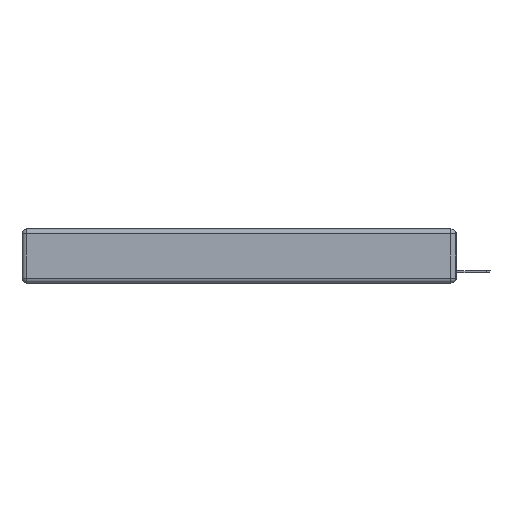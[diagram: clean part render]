
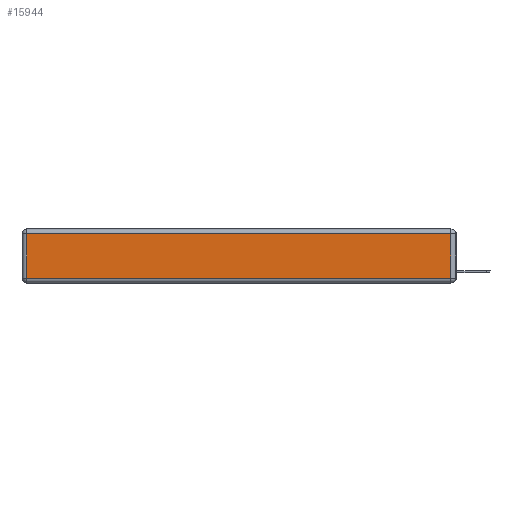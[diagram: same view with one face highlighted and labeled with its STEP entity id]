
A CAD part, left-side view. The second image highlights one B-rep face of the part: STEP entity #15944.
In plain terms, the highlighted planar face has unit normal (-1, 0, 0).
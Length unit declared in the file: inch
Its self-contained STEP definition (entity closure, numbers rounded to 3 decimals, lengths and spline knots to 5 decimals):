
#41 = CARTESIAN_POINT ( 'NONE',  ( 0., 0., -0.343 ) ) ;
#593 = LINE ( 'NONE', #10791, #13308 ) ;
#784 = VERTEX_POINT ( 'NONE', #3760 ) ;
#988 = VECTOR ( 'NONE', #2317, 39.37008 ) ;
#1004 = CARTESIAN_POINT ( 'NONE',  ( 0., 2.72, -0.343 ) ) ;
#2317 = DIRECTION ( 'NONE',  ( 0., 0., -1. ) ) ;
#2895 = EDGE_CURVE ( 'NONE', #784, #14623, #15143, .T. ) ;
#3760 = CARTESIAN_POINT ( 'NONE',  ( 0., 0.03, -0.03 ) ) ;
#4066 = CARTESIAN_POINT ( 'NONE',  ( 0., 0.03, -0.313 ) ) ;
#4266 = DIRECTION ( 'NONE',  ( 0., 0., 1. ) ) ;
#4416 = EDGE_CURVE ( 'NONE', #14623, #6491, #9836, .T. ) ;
#6491 = VERTEX_POINT ( 'NONE', #11413 ) ;
#7182 = VECTOR ( 'NONE', #13332, 39.37008 ) ;
#7221 = DIRECTION ( 'NONE',  ( 0., 0., 1. ) ) ;
#7301 = ORIENTED_EDGE ( 'NONE', *, *, #4416, .T. ) ;
#8003 = CARTESIAN_POINT ( 'NONE',  ( 0., 0.03, -0.343 ) ) ;
#8514 = PLANE ( 'NONE',  #10298 ) ;
#8618 = ORIENTED_EDGE ( 'NONE', *, *, #14991, .T. ) ;
#9686 = ORIENTED_EDGE ( 'NONE', *, *, #2895, .T. ) ;
#9836 = LINE ( 'NONE', #1004, #988 ) ;
#10298 = AXIS2_PLACEMENT_3D ( 'NONE', #41, #14648, #7221 ) ;
#10682 = DIRECTION ( 'NONE',  ( 0., -1., 0. ) ) ;
#10720 = EDGE_LOOP ( 'NONE', ( #14382, #8618, #9686, #7301 ) ) ;
#10767 = CARTESIAN_POINT ( 'NONE',  ( 0., 2.75, -0.03 ) ) ;
#10791 = CARTESIAN_POINT ( 'NONE',  ( 0., 0., -0.313 ) ) ;
#10901 = EDGE_CURVE ( 'NONE', #6491, #14197, #593, .T. ) ;
#11262 = VECTOR ( 'NONE', #4266, 39.37008 ) ;
#11413 = CARTESIAN_POINT ( 'NONE',  ( 0., 2.72, -0.313 ) ) ;
#11701 = FACE_OUTER_BOUND ( 'NONE', #10720, .T. ) ;
#13308 = VECTOR ( 'NONE', #10682, 39.37008 ) ;
#13332 = DIRECTION ( 'NONE',  ( 0., 1., 0. ) ) ;
#13600 = CARTESIAN_POINT ( 'NONE',  ( 0., 2.72, -0.03 ) ) ;
#13823 = LINE ( 'NONE', #8003, #11262 ) ;
#14197 = VERTEX_POINT ( 'NONE', #4066 ) ;
#14382 = ORIENTED_EDGE ( 'NONE', *, *, #10901, .T. ) ;
#14623 = VERTEX_POINT ( 'NONE', #13600 ) ;
#14648 = DIRECTION ( 'NONE',  ( -1., 0., 0. ) ) ;
#14991 = EDGE_CURVE ( 'NONE', #14197, #784, #13823, .T. ) ;
#15143 = LINE ( 'NONE', #10767, #7182 ) ;
#15944 = ADVANCED_FACE ( 'NONE', ( #11701 ), #8514, .T. ) ;
